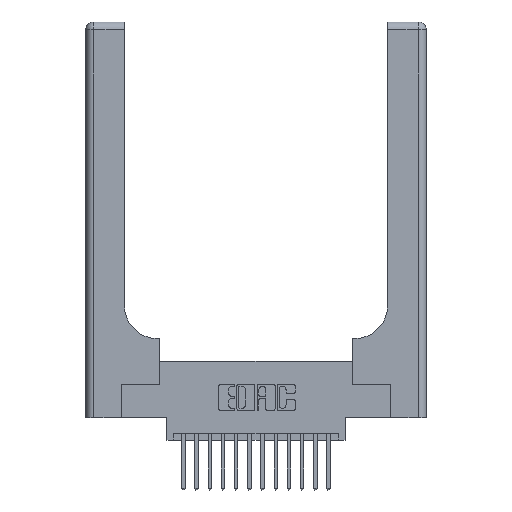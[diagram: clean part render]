
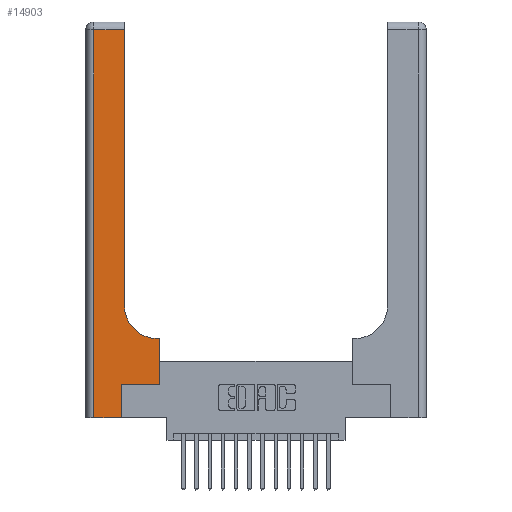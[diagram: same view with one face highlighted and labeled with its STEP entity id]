
A CAD part, top view. The second image highlights one B-rep face of the part: STEP entity #14903.
In plain terms, the highlighted planar face has unit normal (0, 0, 1).
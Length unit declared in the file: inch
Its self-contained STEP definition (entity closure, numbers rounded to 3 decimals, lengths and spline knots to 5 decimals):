
#286 = VECTOR ( 'NONE', #4592, 39.37008 ) ;
#396 = ORIENTED_EDGE ( 'NONE', *, *, #13228, .T. ) ;
#457 = DIRECTION ( 'NONE',  ( 0., 1., 0. ) ) ;
#992 = EDGE_CURVE ( 'NONE', #8211, #10060, #16806, .T. ) ;
#1175 = ORIENTED_EDGE ( 'NONE', *, *, #10347, .T. ) ;
#2181 = DIRECTION ( 'NONE',  ( -1., 0., 0. ) ) ;
#2280 = EDGE_LOOP ( 'NONE', ( #17680, #1175, #10212, #4999, #396, #15707, #13693, #5465, #5075 ) ) ;
#2334 = VERTEX_POINT ( 'NONE', #13386 ) ;
#2456 = DIRECTION ( 'NONE',  ( 0., 0., -1. ) ) ;
#2630 = CARTESIAN_POINT ( 'NONE',  ( 0.5585, 0.25, 0.37 ) ) ;
#3362 = EDGE_CURVE ( 'NONE', #4681, #11576, #11885, .T. ) ;
#3581 = CARTESIAN_POINT ( 'NONE',  ( 0.2915, 0.6, 0.37 ) ) ;
#4042 = FACE_OUTER_BOUND ( 'NONE', #2280, .T. ) ;
#4076 = VECTOR ( 'NONE', #12301, 39.37008 ) ;
#4113 = AXIS2_PLACEMENT_3D ( 'NONE', #18298, #2456, #13914 ) ;
#4487 = LINE ( 'NONE', #12583, #7881 ) ;
#4592 = DIRECTION ( 'NONE',  ( 0., 1., 0. ) ) ;
#4660 = CARTESIAN_POINT ( 'NONE',  ( 0.269, 0., 0.37 ) ) ;
#4681 = VERTEX_POINT ( 'NONE', #6044 ) ;
#4999 = ORIENTED_EDGE ( 'NONE', *, *, #14880, .T. ) ;
#5066 = CARTESIAN_POINT ( 'NONE',  ( 0.5415, 0.6, 0.37 ) ) ;
#5075 = ORIENTED_EDGE ( 'NONE', *, *, #11282, .T. ) ;
#5249 = DIRECTION ( 'NONE',  ( 0., 0., -1. ) ) ;
#5310 = PLANE ( 'NONE',  #9249 ) ;
#5465 = ORIENTED_EDGE ( 'NONE', *, *, #13284, .T. ) ;
#5814 = VERTEX_POINT ( 'NONE', #9843 ) ;
#6044 = CARTESIAN_POINT ( 'NONE',  ( 0.2915, 0.85, 0.37 ) ) ;
#7529 = VECTOR ( 'NONE', #8940, 39.37008 ) ;
#7679 = VECTOR ( 'NONE', #17840, 39.37008 ) ;
#7771 = CARTESIAN_POINT ( 'NONE',  ( 0.269, 0., 0.37 ) ) ;
#7881 = VECTOR ( 'NONE', #15411, 39.37008 ) ;
#8211 = VERTEX_POINT ( 'NONE', #13906 ) ;
#8917 = VECTOR ( 'NONE', #457, 39.37008 ) ;
#8940 = DIRECTION ( 'NONE',  ( -1., 0., 0. ) ) ;
#9029 = EDGE_CURVE ( 'NONE', #13878, #2334, #17199, .T. ) ;
#9031 = DIRECTION ( 'NONE',  ( 0., -1., 0. ) ) ;
#9147 = VERTEX_POINT ( 'NONE', #7771 ) ;
#9249 = AXIS2_PLACEMENT_3D ( 'NONE', #15543, #5249, #2181 ) ;
#9843 = CARTESIAN_POINT ( 'NONE',  ( 0.5585, 0.6, 0.37 ) ) ;
#10060 = VERTEX_POINT ( 'NONE', #2630 ) ;
#10212 = ORIENTED_EDGE ( 'NONE', *, *, #9029, .T. ) ;
#10295 = CIRCLE ( 'NONE', #4113, 0.25 ) ;
#10347 = EDGE_CURVE ( 'NONE', #11576, #13878, #10512, .T. ) ;
#10512 = LINE ( 'NONE', #16113, #7529 ) ;
#10693 = CARTESIAN_POINT ( 'NONE',  ( 0.5585, 0.25, 0.37 ) ) ;
#10872 = DIRECTION ( 'NONE',  ( 1., 0., 0. ) ) ;
#10913 = LINE ( 'NONE', #3581, #4076 ) ;
#11282 = EDGE_CURVE ( 'NONE', #14077, #4681, #10295, .T. ) ;
#11576 = VERTEX_POINT ( 'NONE', #18240 ) ;
#11885 = LINE ( 'NONE', #17914, #8917 ) ;
#11932 = VECTOR ( 'NONE', #9031, 39.37008 ) ;
#12301 = DIRECTION ( 'NONE',  ( -1., 0., 0. ) ) ;
#12583 = CARTESIAN_POINT ( 'NONE',  ( 0., 0., 0.37 ) ) ;
#13228 = EDGE_CURVE ( 'NONE', #9147, #8211, #14367, .T. ) ;
#13284 = EDGE_CURVE ( 'NONE', #5814, #14077, #10913, .T. ) ;
#13386 = CARTESIAN_POINT ( 'NONE',  ( 0.06, 0., 0.37 ) ) ;
#13624 = CARTESIAN_POINT ( 'NONE',  ( 0.06, 2.94, 0.37 ) ) ;
#13693 = ORIENTED_EDGE ( 'NONE', *, *, #18666, .T. ) ;
#13878 = VERTEX_POINT ( 'NONE', #13624 ) ;
#13906 = CARTESIAN_POINT ( 'NONE',  ( 0.269, 0.25, 0.37 ) ) ;
#13914 = DIRECTION ( 'NONE',  ( 1., 0., 0. ) ) ;
#14077 = VERTEX_POINT ( 'NONE', #5066 ) ;
#14367 = LINE ( 'NONE', #4660, #286 ) ;
#14806 = CARTESIAN_POINT ( 'NONE',  ( 0.06, 3., 0.37 ) ) ;
#14880 = EDGE_CURVE ( 'NONE', #2334, #9147, #4487, .T. ) ;
#14903 = ADVANCED_FACE ( 'NONE', ( #4042 ), #5310, .F. ) ;
#15411 = DIRECTION ( 'NONE',  ( 1., 0., 0. ) ) ;
#15543 = CARTESIAN_POINT ( 'NONE',  ( 0., 3., 0.37 ) ) ;
#15707 = ORIENTED_EDGE ( 'NONE', *, *, #992, .T. ) ;
#16113 = CARTESIAN_POINT ( 'NONE',  ( 0., 2.94, 0.37 ) ) ;
#16613 = LINE ( 'NONE', #10693, #7679 ) ;
#16806 = LINE ( 'NONE', #18378, #18392 ) ;
#17199 = LINE ( 'NONE', #14806, #11932 ) ;
#17680 = ORIENTED_EDGE ( 'NONE', *, *, #3362, .T. ) ;
#17840 = DIRECTION ( 'NONE',  ( 0., 1., 0. ) ) ;
#17914 = CARTESIAN_POINT ( 'NONE',  ( 0.2915, 3., 0.37 ) ) ;
#18240 = CARTESIAN_POINT ( 'NONE',  ( 0.2915, 2.94, 0.37 ) ) ;
#18298 = CARTESIAN_POINT ( 'NONE',  ( 0.5415, 0.85, 0.37 ) ) ;
#18378 = CARTESIAN_POINT ( 'NONE',  ( 0.269, 0.25, 0.37 ) ) ;
#18392 = VECTOR ( 'NONE', #10872, 39.37008 ) ;
#18666 = EDGE_CURVE ( 'NONE', #10060, #5814, #16613, .T. ) ;
